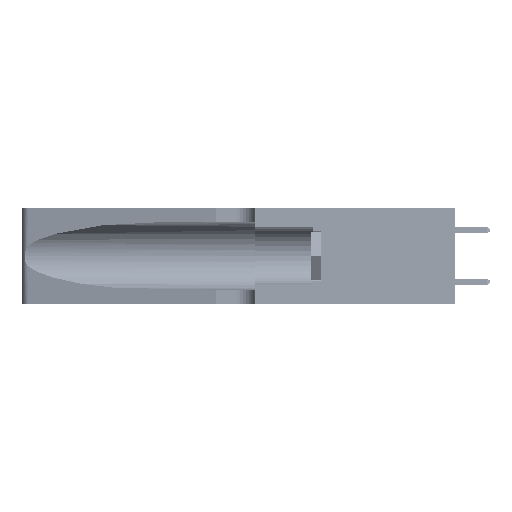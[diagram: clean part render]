
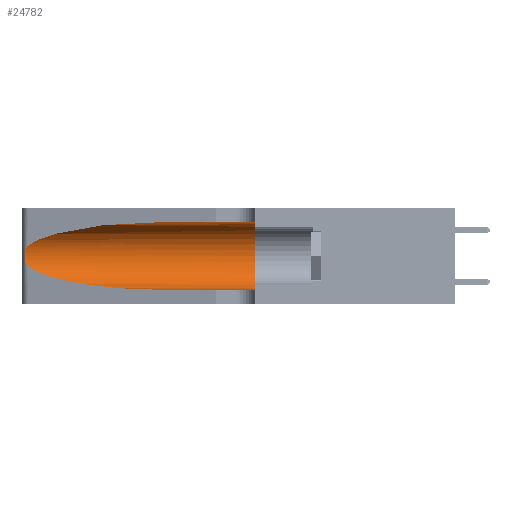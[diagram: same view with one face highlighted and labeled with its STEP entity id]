
A CAD part, left-side view. The second image highlights one B-rep face of the part: STEP entity #24782.
In plain terms, the highlighted cylindrical face has radius 3.308 mm (diameter 6.617 mm), a partial arc.
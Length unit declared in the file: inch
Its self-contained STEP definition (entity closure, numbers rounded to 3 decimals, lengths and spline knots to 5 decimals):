
#236 = CARTESIAN_POINT ( 'NONE',  ( 0.25487, 1.22718, 0.14631 ) ) ;
#1898 = CARTESIAN_POINT ( 'NONE',  ( 0.1305, 1.61858, 0.185 ) ) ;
#2687 = LINE ( 'NONE', #41484, #31313 ) ;
#4963 = EDGE_CURVE ( 'NONE', #19257, #13884, #32099, .T. ) ;
#5216 =( BOUNDED_CURVE ( )  B_SPLINE_CURVE ( 3, ( #8282, #16151, #42256, #41920 ),
 .UNSPECIFIED., .F., .T. ) 
 B_SPLINE_CURVE_WITH_KNOTS ( ( 4, 4 ),
 ( 3.44316, 4.71239 ),
 .UNSPECIFIED. ) 
 CURVE ( )  GEOMETRIC_REPRESENTATION_ITEM ( )  RATIONAL_B_SPLINE_CURVE ( ( 1., 0.87, 0.87, 1. ) ) 
 REPRESENTATION_ITEM ( '' )  );
#6258 = EDGE_CURVE ( 'NONE', #10733, #19257, #5216, .T. ) ;
#6490 = CARTESIAN_POINT ( 'NONE',  ( 0.25639, 1.23186, 0.15144 ) ) ;
#6698 = CARTESIAN_POINT ( 'NONE',  ( 0.25487, 1.22718, 0.22369 ) ) ;
#7899 = CARTESIAN_POINT ( 'NONE',  ( 0.1305, 0.72297, 0.05475 ) ) ;
#7967 = AXIS2_PLACEMENT_3D ( 'NONE', #15543, #41659, #26950 ) ;
#8282 = CARTESIAN_POINT ( 'NONE',  ( 0.25487, 1.22718, 0.14631 ) ) ;
#10070 = CARTESIAN_POINT ( 'NONE',  ( 0.26075, 1.23896, 0.178 ) ) ;
#10733 = VERTEX_POINT ( 'NONE', #236 ) ;
#12994 = DIRECTION ( 'NONE',  ( 0., -1., 0. ) ) ;
#13520 = CARTESIAN_POINT ( 'NONE',  ( 0.25555, 1.22994, 0.2215 ) ) ;
#13884 = VERTEX_POINT ( 'NONE', #46608 ) ;
#14936 = EDGE_LOOP ( 'NONE', ( #42960, #16704, #25066, #45018, #28487, #41266 ) ) ;
#14985 = CIRCLE ( 'NONE', #7967, 0.13025 ) ;
#15543 = CARTESIAN_POINT ( 'NONE',  ( 0.1305, 0.35, 0.185 ) ) ;
#15599 = DIRECTION ( 'NONE',  ( 0., -1., 0. ) ) ;
#16151 = CARTESIAN_POINT ( 'NONE',  ( 0.2373, 1.15595, 0.08982 ) ) ;
#16704 = ORIENTED_EDGE ( 'NONE', *, *, #18524, .T. ) ;
#17118 = CYLINDRICAL_SURFACE ( 'NONE', #27383, 0.13025 ) ;
#17448 = CARTESIAN_POINT ( 'NONE',  ( 0.25854, 1.2359, 0.20912 ) ) ;
#18524 = EDGE_CURVE ( 'NONE', #26177, #10733, #41396, .T. ) ;
#19257 = VERTEX_POINT ( 'NONE', #7899 ) ;
#20020 = FACE_OUTER_BOUND ( 'NONE', #14936, .T. ) ;
#21346 = CARTESIAN_POINT ( 'NONE',  ( 0.25487, 1.22718, 0.22369 ) ) ;
#21496 = CARTESIAN_POINT ( 'NONE',  ( 0.26075, 1.23896, 0.19203 ) ) ;
#22767 = VECTOR ( 'NONE', #15599, 39.37008 ) ;
#24125 = VERTEX_POINT ( 'NONE', #33323 ) ;
#24782 = ADVANCED_FACE ( 'NONE', ( #20020 ), #17118, .F. ) ;
#25066 = ORIENTED_EDGE ( 'NONE', *, *, #6258, .T. ) ;
#25224 = CARTESIAN_POINT ( 'NONE',  ( 0.25555, 1.22993, 0.14849 ) ) ;
#25267 = CARTESIAN_POINT ( 'NONE',  ( 0.2373, 1.15595, 0.28018 ) ) ;
#25381 = CARTESIAN_POINT ( 'NONE',  ( 0.25789, 1.23486, 0.15765 ) ) ;
#26177 = VERTEX_POINT ( 'NONE', #39951 ) ;
#26950 = DIRECTION ( 'NONE',  ( 0., 0., 1. ) ) ;
#27027 =( BOUNDED_CURVE ( )  B_SPLINE_CURVE ( 3, ( #39995, #28915, #25267, #6698 ),
 .UNSPECIFIED., .F., .F. ) 
 B_SPLINE_CURVE_WITH_KNOTS ( ( 4, 4 ),
 ( 1.5708, 2.84003 ),
 .UNSPECIFIED. ) 
 CURVE ( )  GEOMETRIC_REPRESENTATION_ITEM ( )  RATIONAL_B_SPLINE_CURVE ( ( 1., 0.87, 0.87, 1. ) ) 
 REPRESENTATION_ITEM ( '' )  );
#27383 = AXIS2_PLACEMENT_3D ( 'NONE', #1898, #12994, #39093 ) ;
#28469 = EDGE_CURVE ( 'NONE', #24125, #26177, #27027, .T. ) ;
#28487 = ORIENTED_EDGE ( 'NONE', *, *, #46507, .F. ) ;
#28536 = CARTESIAN_POINT ( 'NONE',  ( 0.25787, 1.23484, 0.2124 ) ) ;
#28870 = CARTESIAN_POINT ( 'NONE',  ( 0.26018, 1.23835, 0.19895 ) ) ;
#28915 = CARTESIAN_POINT ( 'NONE',  ( 0.18966, 0.96281, 0.31525 ) ) ;
#29968 = EDGE_CURVE ( 'NONE', #24125, #30868, #2687, .T. ) ;
#30868 = VERTEX_POINT ( 'NONE', #39882 ) ;
#31313 = VECTOR ( 'NONE', #37583, 39.37008 ) ;
#32099 = LINE ( 'NONE', #33890, #22767 ) ;
#32755 = CARTESIAN_POINT ( 'NONE',  ( 0.26017, 1.23833, 0.17102 ) ) ;
#33076 = CARTESIAN_POINT ( 'NONE',  ( 0.25487, 1.22718, 0.14631 ) ) ;
#33323 = CARTESIAN_POINT ( 'NONE',  ( 0.1305, 0.72297, 0.31525 ) ) ;
#33890 = CARTESIAN_POINT ( 'NONE',  ( 0.1305, 1.61858, 0.05475 ) ) ;
#37583 = DIRECTION ( 'NONE',  ( 0., -1., 0. ) ) ;
#39093 = DIRECTION ( 'NONE',  ( 0., 0., -1. ) ) ;
#39882 = CARTESIAN_POINT ( 'NONE',  ( 0.1305, 0.35, 0.31525 ) ) ;
#39951 = CARTESIAN_POINT ( 'NONE',  ( 0.25487, 1.22718, 0.22369 ) ) ;
#39995 = CARTESIAN_POINT ( 'NONE',  ( 0.1305, 0.72297, 0.31525 ) ) ;
#41266 = ORIENTED_EDGE ( 'NONE', *, *, #29968, .F. ) ;
#41396 = B_SPLINE_CURVE_WITH_KNOTS ( 'NONE', 3,
 ( #21346, #13520, #47762, #28536, #17448, #28870, #21496, #10070, #32755, #47603, #25381, #6490, #25224, #33076 ),
 .UNSPECIFIED., .F., .F.,
 ( 4, 2, 2, 2, 2, 2, 4 ),
 ( 0., 0.00027, 0.00053, 0.00107, 0.0016, 0.00187, 0.00214 ),
 .UNSPECIFIED. ) ;
#41484 = CARTESIAN_POINT ( 'NONE',  ( 0.1305, 1.61858, 0.31525 ) ) ;
#41659 = DIRECTION ( 'NONE',  ( 0., 1., 0. ) ) ;
#41920 = CARTESIAN_POINT ( 'NONE',  ( 0.1305, 0.72297, 0.05475 ) ) ;
#42256 = CARTESIAN_POINT ( 'NONE',  ( 0.18966, 0.96281, 0.05475 ) ) ;
#42960 = ORIENTED_EDGE ( 'NONE', *, *, #28469, .T. ) ;
#45018 = ORIENTED_EDGE ( 'NONE', *, *, #4963, .T. ) ;
#46507 = EDGE_CURVE ( 'NONE', #30868, #13884, #14985, .T. ) ;
#46608 = CARTESIAN_POINT ( 'NONE',  ( 0.1305, 0.35, 0.05475 ) ) ;
#47603 = CARTESIAN_POINT ( 'NONE',  ( 0.25856, 1.23593, 0.16098 ) ) ;
#47762 = CARTESIAN_POINT ( 'NONE',  ( 0.25639, 1.23184, 0.21858 ) ) ;
